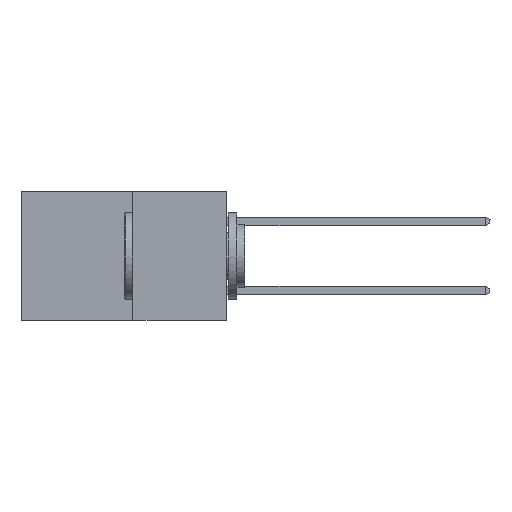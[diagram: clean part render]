
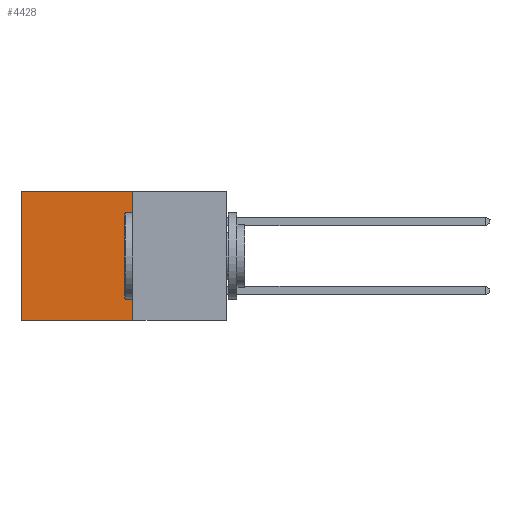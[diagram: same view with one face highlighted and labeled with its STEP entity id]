
A CAD part, left-side view. The second image highlights one B-rep face of the part: STEP entity #4428.
In plain terms, the highlighted planar face has unit normal (-1, 0, 0).
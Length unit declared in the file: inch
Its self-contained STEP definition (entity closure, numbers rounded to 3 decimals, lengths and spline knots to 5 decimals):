
#1244 = DIRECTION ( 'NONE',  ( 0., 0., -1. ) ) ;
#1759 = EDGE_CURVE ( 'NONE', #17271, #15084, #14221, .T. ) ;
#2911 = LINE ( 'NONE', #10324, #12122 ) ;
#2916 = DIRECTION ( 'NONE',  ( 0., 1., 0. ) ) ;
#4070 = EDGE_LOOP ( 'NONE', ( #11256, #20919, #20944, #11694 ) ) ;
#4424 = CARTESIAN_POINT ( 'NONE',  ( 0.277, 0.59, 0. ) ) ;
#4428 = ADVANCED_FACE ( 'NONE', ( #19108 ), #6014, .F. ) ;
#5502 = DIRECTION ( 'NONE',  ( 0., 0., -1. ) ) ;
#5768 = DIRECTION ( 'NONE',  ( 1., 0., 0. ) ) ;
#6014 = PLANE ( 'NONE',  #9090 ) ;
#6372 = EDGE_CURVE ( 'NONE', #15726, #15084, #22518, .T. ) ;
#7027 = CARTESIAN_POINT ( 'NONE',  ( 0.277, 0.27, -0.37 ) ) ;
#7641 = CARTESIAN_POINT ( 'NONE',  ( 0.277, 0.27, -0.37 ) ) ;
#8825 = CARTESIAN_POINT ( 'NONE',  ( 0.277, 0.27, 0. ) ) ;
#9090 = AXIS2_PLACEMENT_3D ( 'NONE', #7641, #5768, #5502 ) ;
#9448 = VECTOR ( 'NONE', #10773, 39.37008 ) ;
#10324 = CARTESIAN_POINT ( 'NONE',  ( 0.277, 0.27, 0. ) ) ;
#10345 = EDGE_CURVE ( 'NONE', #22951, #15726, #2911, .T. ) ;
#10445 = CARTESIAN_POINT ( 'NONE',  ( 0.277, 0.27, -0.37 ) ) ;
#10773 = DIRECTION ( 'NONE',  ( 0., 1., 0. ) ) ;
#11256 = ORIENTED_EDGE ( 'NONE', *, *, #6372, .T. ) ;
#11694 = ORIENTED_EDGE ( 'NONE', *, *, #10345, .T. ) ;
#11851 = CARTESIAN_POINT ( 'NONE',  ( 0.277, 0.59, -0.37 ) ) ;
#12122 = VECTOR ( 'NONE', #2916, 39.37008 ) ;
#12428 = VECTOR ( 'NONE', #1244, 39.37008 ) ;
#13166 = VECTOR ( 'NONE', #21306, 39.37008 ) ;
#14221 = LINE ( 'NONE', #7027, #9448 ) ;
#15084 = VERTEX_POINT ( 'NONE', #11851 ) ;
#15726 = VERTEX_POINT ( 'NONE', #4424 ) ;
#17096 = CARTESIAN_POINT ( 'NONE',  ( 0.277, 0.27, -0.37 ) ) ;
#17271 = VERTEX_POINT ( 'NONE', #17096 ) ;
#19044 = CARTESIAN_POINT ( 'NONE',  ( 0.277, 0.59, -0.37 ) ) ;
#19108 = FACE_OUTER_BOUND ( 'NONE', #4070, .T. ) ;
#20919 = ORIENTED_EDGE ( 'NONE', *, *, #1759, .F. ) ;
#20944 = ORIENTED_EDGE ( 'NONE', *, *, #21965, .F. ) ;
#21306 = DIRECTION ( 'NONE',  ( 0., 0., -1. ) ) ;
#21965 = EDGE_CURVE ( 'NONE', #22951, #17271, #22335, .T. ) ;
#22335 = LINE ( 'NONE', #10445, #12428 ) ;
#22518 = LINE ( 'NONE', #19044, #13166 ) ;
#22951 = VERTEX_POINT ( 'NONE', #8825 ) ;
